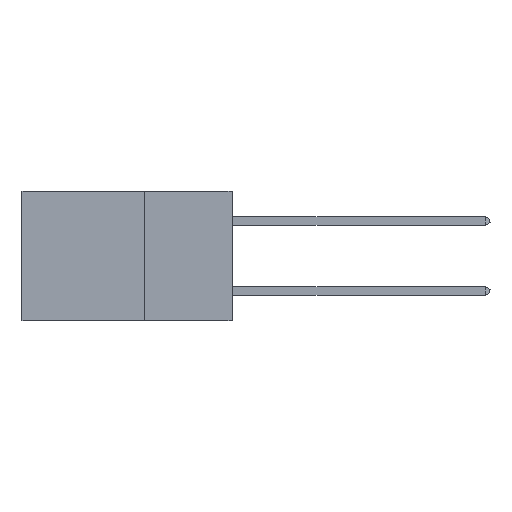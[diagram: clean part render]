
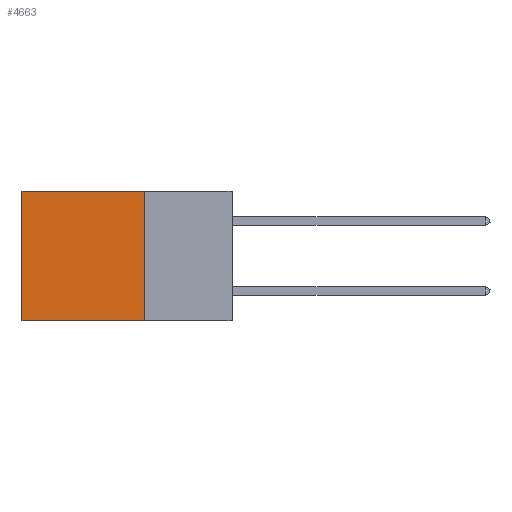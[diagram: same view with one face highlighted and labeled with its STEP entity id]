
A CAD part, left-side view. The second image highlights one B-rep face of the part: STEP entity #4663.
In plain terms, the highlighted planar face has unit normal (-1, 0, 0).
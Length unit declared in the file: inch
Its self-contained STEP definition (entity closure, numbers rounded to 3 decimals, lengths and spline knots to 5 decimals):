
#146 = VERTEX_POINT ( 'NONE', #17958 ) ;
#1215 = VECTOR ( 'NONE', #4671, 39.37008 ) ;
#1295 = VECTOR ( 'NONE', #8705, 39.37008 ) ;
#1460 = ORIENTED_EDGE ( 'NONE', *, *, #19023, .F. ) ;
#1958 = FACE_OUTER_BOUND ( 'NONE', #4725, .T. ) ;
#2381 = EDGE_CURVE ( 'NONE', #12808, #146, #8110, .T. ) ;
#3911 = VERTEX_POINT ( 'NONE', #20454 ) ;
#4568 = CARTESIAN_POINT ( 'NONE',  ( 0.2875, 0.25, 0. ) ) ;
#4663 = ADVANCED_FACE ( 'NONE', ( #1958 ), #12844, .F. ) ;
#4671 = DIRECTION ( 'NONE',  ( 0., 1., 0. ) ) ;
#4725 = EDGE_LOOP ( 'NONE', ( #11896, #1460, #6305, #19818 ) ) ;
#6305 = ORIENTED_EDGE ( 'NONE', *, *, #14005, .F. ) ;
#8110 = LINE ( 'NONE', #19515, #1215 ) ;
#8464 = CARTESIAN_POINT ( 'NONE',  ( 0.2875, 0.6, 0. ) ) ;
#8625 = CARTESIAN_POINT ( 'NONE',  ( 0.2875, 0.25, 0. ) ) ;
#8705 = DIRECTION ( 'NONE',  ( 0., 0., -1. ) ) ;
#8862 = AXIS2_PLACEMENT_3D ( 'NONE', #13078, #16815, #9304 ) ;
#9304 = DIRECTION ( 'NONE',  ( 0., 0., -1. ) ) ;
#11896 = ORIENTED_EDGE ( 'NONE', *, *, #21291, .T. ) ;
#12808 = VERTEX_POINT ( 'NONE', #8625 ) ;
#12844 = PLANE ( 'NONE',  #8862 ) ;
#13078 = CARTESIAN_POINT ( 'NONE',  ( 0.2875, 0.25, 0. ) ) ;
#13441 = DIRECTION ( 'NONE',  ( 0., 0., -1. ) ) ;
#14005 = EDGE_CURVE ( 'NONE', #12808, #19730, #19892, .T. ) ;
#14374 = LINE ( 'NONE', #18827, #21894 ) ;
#16104 = CARTESIAN_POINT ( 'NONE',  ( 0.2875, 0.25, -0.37 ) ) ;
#16558 = DIRECTION ( 'NONE',  ( 0., 1., 0. ) ) ;
#16815 = DIRECTION ( 'NONE',  ( 1., 0., 0. ) ) ;
#17958 = CARTESIAN_POINT ( 'NONE',  ( 0.2875, 0.6, 0. ) ) ;
#18827 = CARTESIAN_POINT ( 'NONE',  ( 0.2875, 0.25, -0.37 ) ) ;
#19023 = EDGE_CURVE ( 'NONE', #19730, #3911, #14374, .T. ) ;
#19515 = CARTESIAN_POINT ( 'NONE',  ( 0.2875, 0.25, 0. ) ) ;
#19730 = VERTEX_POINT ( 'NONE', #16104 ) ;
#19797 = LINE ( 'NONE', #8464, #1295 ) ;
#19818 = ORIENTED_EDGE ( 'NONE', *, *, #2381, .T. ) ;
#19892 = LINE ( 'NONE', #4568, #20186 ) ;
#20186 = VECTOR ( 'NONE', #13441, 39.37008 ) ;
#20454 = CARTESIAN_POINT ( 'NONE',  ( 0.2875, 0.6, -0.37 ) ) ;
#21291 = EDGE_CURVE ( 'NONE', #146, #3911, #19797, .T. ) ;
#21894 = VECTOR ( 'NONE', #16558, 39.37008 ) ;
